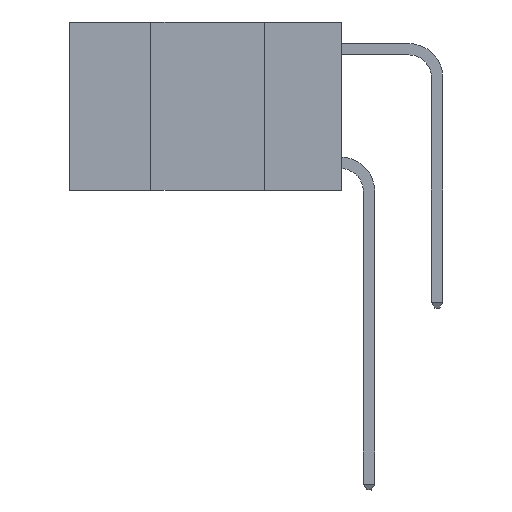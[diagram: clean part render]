
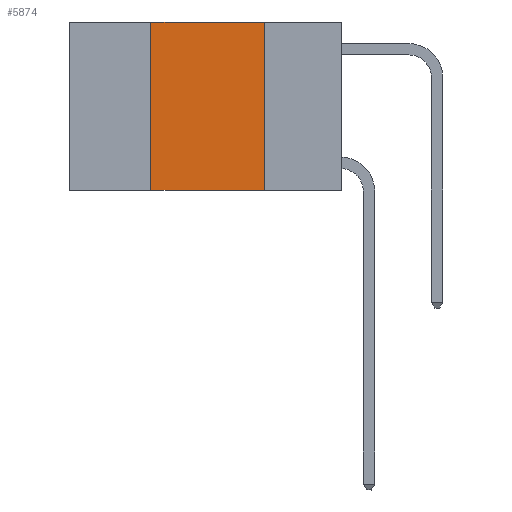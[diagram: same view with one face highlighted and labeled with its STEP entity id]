
A CAD part, left-side view. The second image highlights one B-rep face of the part: STEP entity #5874.
In plain terms, the highlighted planar face has unit normal (-1, 0, 0).
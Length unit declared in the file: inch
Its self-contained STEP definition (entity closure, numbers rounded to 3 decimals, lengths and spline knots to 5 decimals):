
#897 = VERTEX_POINT ( 'NONE', #9723 ) ;
#1137 = EDGE_CURVE ( 'NONE', #897, #10920, #15490, .T. ) ;
#1240 = ORIENTED_EDGE ( 'NONE', *, *, #9399, .F. ) ;
#1595 = VECTOR ( 'NONE', #13684, 39.37008 ) ;
#1627 = CARTESIAN_POINT ( 'NONE',  ( 0., 0.42, 0. ) ) ;
#2678 = LINE ( 'NONE', #21483, #7949 ) ;
#2803 = ORIENTED_EDGE ( 'NONE', *, *, #22053, .F. ) ;
#3551 = EDGE_CURVE ( 'NONE', #897, #13215, #9064, .T. ) ;
#4432 = CARTESIAN_POINT ( 'NONE',  ( 0., 0.6, 0. ) ) ;
#5874 = ADVANCED_FACE ( 'NONE', ( #13514 ), #13041, .F. ) ;
#6493 = AXIS2_PLACEMENT_3D ( 'NONE', #4432, #20041, #9684 ) ;
#6749 = LINE ( 'NONE', #9185, #15314 ) ;
#6894 = CARTESIAN_POINT ( 'NONE',  ( 0., 0.6, -0.37 ) ) ;
#7949 = VECTOR ( 'NONE', #12800, 39.37008 ) ;
#9064 = LINE ( 'NONE', #1627, #18776 ) ;
#9185 = CARTESIAN_POINT ( 'NONE',  ( 0., 0.17, 0. ) ) ;
#9399 = EDGE_CURVE ( 'NONE', #19141, #10920, #6749, .T. ) ;
#9684 = DIRECTION ( 'NONE',  ( 0., 0., -1. ) ) ;
#9723 = CARTESIAN_POINT ( 'NONE',  ( 0., 0.42, -0.37 ) ) ;
#10920 = VERTEX_POINT ( 'NONE', #16968 ) ;
#12800 = DIRECTION ( 'NONE',  ( 0., -1., 0. ) ) ;
#13041 = PLANE ( 'NONE',  #6493 ) ;
#13138 = CARTESIAN_POINT ( 'NONE',  ( 0., 0.42, 0. ) ) ;
#13215 = VERTEX_POINT ( 'NONE', #13138 ) ;
#13514 = FACE_OUTER_BOUND ( 'NONE', #16723, .T. ) ;
#13684 = DIRECTION ( 'NONE',  ( 0., -1., 0. ) ) ;
#14352 = DIRECTION ( 'NONE',  ( 0., 0., -1. ) ) ;
#15314 = VECTOR ( 'NONE', #14352, 39.37008 ) ;
#15490 = LINE ( 'NONE', #6894, #1595 ) ;
#16723 = EDGE_LOOP ( 'NONE', ( #1240, #2803, #18028, #19440 ) ) ;
#16968 = CARTESIAN_POINT ( 'NONE',  ( 0., 0.17, -0.37 ) ) ;
#17306 = DIRECTION ( 'NONE',  ( 0., 0., 1. ) ) ;
#18028 = ORIENTED_EDGE ( 'NONE', *, *, #3551, .F. ) ;
#18776 = VECTOR ( 'NONE', #17306, 39.37008 ) ;
#19141 = VERTEX_POINT ( 'NONE', #22475 ) ;
#19440 = ORIENTED_EDGE ( 'NONE', *, *, #1137, .T. ) ;
#20041 = DIRECTION ( 'NONE',  ( 1., 0., 0. ) ) ;
#21483 = CARTESIAN_POINT ( 'NONE',  ( 0., 0.6, 0. ) ) ;
#22053 = EDGE_CURVE ( 'NONE', #13215, #19141, #2678, .T. ) ;
#22475 = CARTESIAN_POINT ( 'NONE',  ( 0., 0.17, 0. ) ) ;
